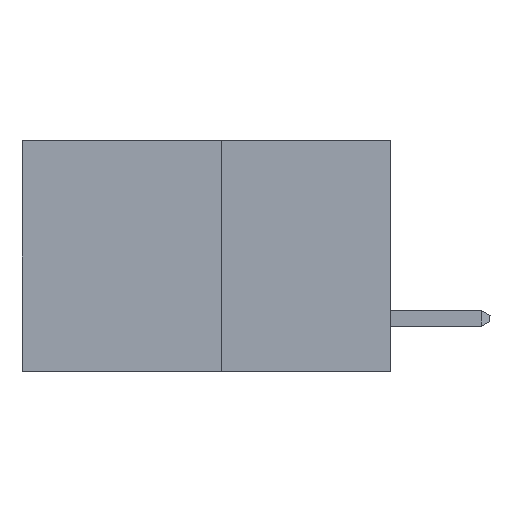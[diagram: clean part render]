
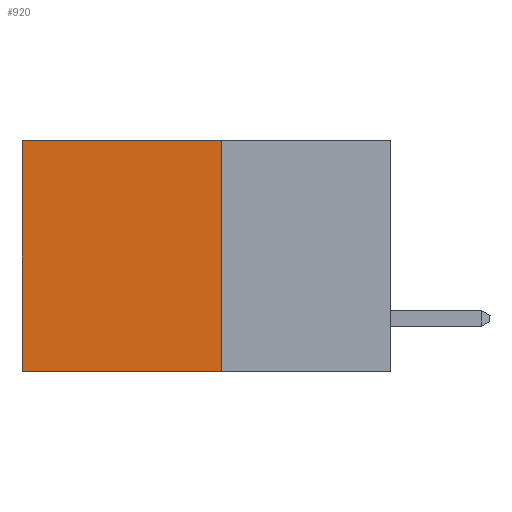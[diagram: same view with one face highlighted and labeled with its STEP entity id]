
A CAD part, left-side view. The second image highlights one B-rep face of the part: STEP entity #920.
In plain terms, the highlighted planar face has unit normal (-1, 0, 0).
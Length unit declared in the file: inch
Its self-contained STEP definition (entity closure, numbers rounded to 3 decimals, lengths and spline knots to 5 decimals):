
#651 = CARTESIAN_POINT ( 'NONE',  ( 0.277, 0.27, -0.37 ) ) ;
#687 = EDGE_CURVE ( 'NONE', #9542, #8724, #9126, .T. ) ;
#920 = ADVANCED_FACE ( 'NONE', ( #6271 ), #10729, .F. ) ;
#1902 = VECTOR ( 'NONE', #9417, 39.37008 ) ;
#2454 = ORIENTED_EDGE ( 'NONE', *, *, #687, .F. ) ;
#3113 = VERTEX_POINT ( 'NONE', #6341 ) ;
#3432 = CARTESIAN_POINT ( 'NONE',  ( 0.277, 0.27, -0.37 ) ) ;
#3975 = DIRECTION ( 'NONE',  ( 0., 1., 0. ) ) ;
#4279 = LINE ( 'NONE', #8663, #8948 ) ;
#4477 = CARTESIAN_POINT ( 'NONE',  ( 0.277, 0.27, -0.37 ) ) ;
#4683 = VECTOR ( 'NONE', #5394, 39.37008 ) ;
#4869 = EDGE_CURVE ( 'NONE', #3113, #8724, #11176, .T. ) ;
#4976 = AXIS2_PLACEMENT_3D ( 'NONE', #651, #6759, #7804 ) ;
#5123 = EDGE_CURVE ( 'NONE', #11841, #3113, #4279, .T. ) ;
#5394 = DIRECTION ( 'NONE',  ( 0., 0., -1. ) ) ;
#5663 = EDGE_LOOP ( 'NONE', ( #8107, #2454, #7449, #10983 ) ) ;
#5711 = CARTESIAN_POINT ( 'NONE',  ( 0.277, 0.59, -0.37 ) ) ;
#5740 = CARTESIAN_POINT ( 'NONE',  ( 0.277, 0.27, 0. ) ) ;
#6271 = FACE_OUTER_BOUND ( 'NONE', #5663, .T. ) ;
#6341 = CARTESIAN_POINT ( 'NONE',  ( 0.277, 0.59, 0. ) ) ;
#6759 = DIRECTION ( 'NONE',  ( 1., 0., 0. ) ) ;
#7324 = EDGE_CURVE ( 'NONE', #11841, #9542, #11962, .T. ) ;
#7389 = CARTESIAN_POINT ( 'NONE',  ( 0.277, 0.59, -0.37 ) ) ;
#7449 = ORIENTED_EDGE ( 'NONE', *, *, #7324, .F. ) ;
#7804 = DIRECTION ( 'NONE',  ( 0., 0., -1. ) ) ;
#8107 = ORIENTED_EDGE ( 'NONE', *, *, #4869, .T. ) ;
#8309 = DIRECTION ( 'NONE',  ( 0., 0., -1. ) ) ;
#8663 = CARTESIAN_POINT ( 'NONE',  ( 0.277, 0.27, 0. ) ) ;
#8724 = VERTEX_POINT ( 'NONE', #5711 ) ;
#8814 = VECTOR ( 'NONE', #8309, 39.37008 ) ;
#8948 = VECTOR ( 'NONE', #3975, 39.37008 ) ;
#9126 = LINE ( 'NONE', #10374, #1902 ) ;
#9417 = DIRECTION ( 'NONE',  ( 0., 1., 0. ) ) ;
#9542 = VERTEX_POINT ( 'NONE', #4477 ) ;
#10374 = CARTESIAN_POINT ( 'NONE',  ( 0.277, 0.27, -0.37 ) ) ;
#10729 = PLANE ( 'NONE',  #4976 ) ;
#10983 = ORIENTED_EDGE ( 'NONE', *, *, #5123, .T. ) ;
#11176 = LINE ( 'NONE', #7389, #8814 ) ;
#11841 = VERTEX_POINT ( 'NONE', #5740 ) ;
#11962 = LINE ( 'NONE', #3432, #4683 ) ;
